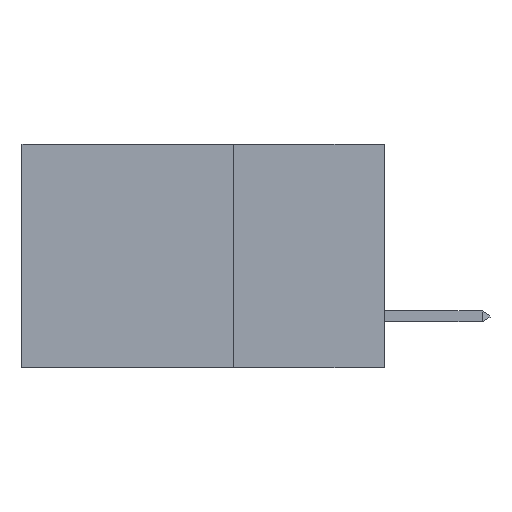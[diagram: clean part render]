
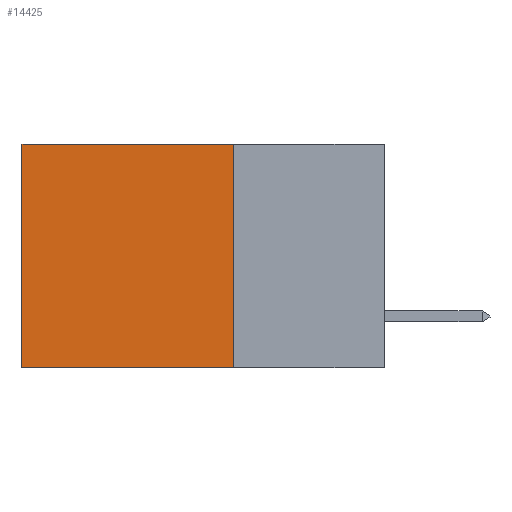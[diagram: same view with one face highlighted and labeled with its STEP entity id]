
A CAD part, left-side view. The second image highlights one B-rep face of the part: STEP entity #14425.
In plain terms, the highlighted planar face has unit normal (-1, 0, 0).
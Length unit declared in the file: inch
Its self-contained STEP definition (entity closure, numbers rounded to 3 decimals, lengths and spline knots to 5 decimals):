
#393 = CARTESIAN_POINT ( 'NONE',  ( 0.2875, 0.25, 0. ) ) ;
#1388 = VECTOR ( 'NONE', #22902, 39.37008 ) ;
#1699 = VECTOR ( 'NONE', #11541, 39.37008 ) ;
#2737 = FACE_OUTER_BOUND ( 'NONE', #13561, .T. ) ;
#3028 = DIRECTION ( 'NONE',  ( 0., 0., -1. ) ) ;
#3920 = VERTEX_POINT ( 'NONE', #30633 ) ;
#4107 = CARTESIAN_POINT ( 'NONE',  ( 0.2875, 0.25, 0. ) ) ;
#4699 = CARTESIAN_POINT ( 'NONE',  ( 0.2875, 0.25, 0. ) ) ;
#6007 = CARTESIAN_POINT ( 'NONE',  ( 0.2875, 0.25, 0. ) ) ;
#7024 = ORIENTED_EDGE ( 'NONE', *, *, #13019, .F. ) ;
#7332 = DIRECTION ( 'NONE',  ( 0., 1., 0. ) ) ;
#7717 = VECTOR ( 'NONE', #3028, 39.37008 ) ;
#8151 = ORIENTED_EDGE ( 'NONE', *, *, #30412, .T. ) ;
#8614 = DIRECTION ( 'NONE',  ( 1., 0., 0. ) ) ;
#8619 = LINE ( 'NONE', #8906, #1699 ) ;
#8906 = CARTESIAN_POINT ( 'NONE',  ( 0.2875, 0.25, -0.37 ) ) ;
#9963 = CARTESIAN_POINT ( 'NONE',  ( 0.2875, 0.6, 0. ) ) ;
#11062 = EDGE_CURVE ( 'NONE', #3920, #24167, #8619, .T. ) ;
#11541 = DIRECTION ( 'NONE',  ( 0., 1., 0. ) ) ;
#12193 = CARTESIAN_POINT ( 'NONE',  ( 0.2875, 0.6, 0. ) ) ;
#13019 = EDGE_CURVE ( 'NONE', #17508, #3920, #14616, .T. ) ;
#13561 = EDGE_LOOP ( 'NONE', ( #8151, #20123, #7024, #25343 ) ) ;
#14425 = ADVANCED_FACE ( 'NONE', ( #2737 ), #21564, .F. ) ;
#14616 = LINE ( 'NONE', #393, #7717 ) ;
#14749 = LINE ( 'NONE', #4699, #20861 ) ;
#15848 = CARTESIAN_POINT ( 'NONE',  ( 0.2875, 0.6, -0.37 ) ) ;
#16191 = AXIS2_PLACEMENT_3D ( 'NONE', #6007, #8614, #26806 ) ;
#17508 = VERTEX_POINT ( 'NONE', #4107 ) ;
#17574 = VERTEX_POINT ( 'NONE', #12193 ) ;
#20123 = ORIENTED_EDGE ( 'NONE', *, *, #11062, .F. ) ;
#20861 = VECTOR ( 'NONE', #7332, 39.37008 ) ;
#21564 = PLANE ( 'NONE',  #16191 ) ;
#22902 = DIRECTION ( 'NONE',  ( 0., 0., -1. ) ) ;
#24167 = VERTEX_POINT ( 'NONE', #15848 ) ;
#25343 = ORIENTED_EDGE ( 'NONE', *, *, #31043, .T. ) ;
#26806 = DIRECTION ( 'NONE',  ( 0., 0., -1. ) ) ;
#29062 = LINE ( 'NONE', #9963, #1388 ) ;
#30412 = EDGE_CURVE ( 'NONE', #17574, #24167, #29062, .T. ) ;
#30633 = CARTESIAN_POINT ( 'NONE',  ( 0.2875, 0.25, -0.37 ) ) ;
#31043 = EDGE_CURVE ( 'NONE', #17508, #17574, #14749, .T. ) ;
